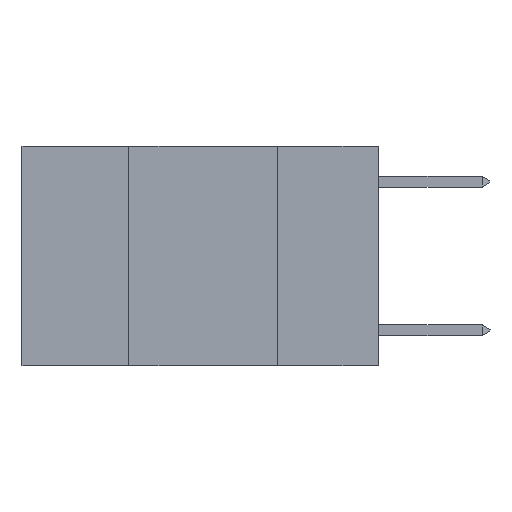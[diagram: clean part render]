
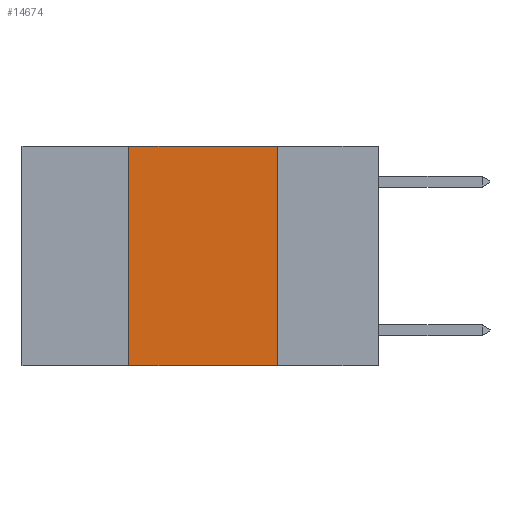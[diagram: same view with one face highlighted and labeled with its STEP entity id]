
A CAD part, left-side view. The second image highlights one B-rep face of the part: STEP entity #14674.
In plain terms, the highlighted planar face has unit normal (-1, 0, 0).
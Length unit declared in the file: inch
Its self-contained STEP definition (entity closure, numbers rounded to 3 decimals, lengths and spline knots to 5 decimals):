
#2302 = ORIENTED_EDGE ( 'NONE', *, *, #11323, .F. ) ;
#2516 = CARTESIAN_POINT ( 'NONE',  ( 0., 0.42, -0.37 ) ) ;
#2889 = VECTOR ( 'NONE', #8701, 39.37008 ) ;
#4548 = EDGE_CURVE ( 'NONE', #9651, #17047, #11353, .T. ) ;
#4781 = VECTOR ( 'NONE', #13084, 39.37008 ) ;
#5238 = DIRECTION ( 'NONE',  ( 0., 0., -1. ) ) ;
#6014 = EDGE_CURVE ( 'NONE', #7529, #14678, #7711, .T. ) ;
#6835 = CARTESIAN_POINT ( 'NONE',  ( 0., 0.17, -0.37 ) ) ;
#6923 = CARTESIAN_POINT ( 'NONE',  ( 0., 0.6, -0.37 ) ) ;
#7529 = VERTEX_POINT ( 'NONE', #2516 ) ;
#7711 = LINE ( 'NONE', #7807, #16832 ) ;
#7807 = CARTESIAN_POINT ( 'NONE',  ( 0., 0.42, 0. ) ) ;
#8701 = DIRECTION ( 'NONE',  ( 0., -1., 0. ) ) ;
#8879 = ORIENTED_EDGE ( 'NONE', *, *, #4548, .F. ) ;
#9391 = EDGE_CURVE ( 'NONE', #7529, #17047, #17040, .T. ) ;
#9634 = EDGE_LOOP ( 'NONE', ( #8879, #2302, #17890, #10650 ) ) ;
#9651 = VERTEX_POINT ( 'NONE', #10568 ) ;
#9659 = VECTOR ( 'NONE', #9911, 39.37008 ) ;
#9813 = CARTESIAN_POINT ( 'NONE',  ( 0., 0.17, 0. ) ) ;
#9911 = DIRECTION ( 'NONE',  ( 0., -1., 0. ) ) ;
#10568 = CARTESIAN_POINT ( 'NONE',  ( 0., 0.17, 0. ) ) ;
#10650 = ORIENTED_EDGE ( 'NONE', *, *, #9391, .T. ) ;
#10736 = FACE_OUTER_BOUND ( 'NONE', #9634, .T. ) ;
#11323 = EDGE_CURVE ( 'NONE', #14678, #9651, #11979, .T. ) ;
#11353 = LINE ( 'NONE', #9813, #4781 ) ;
#11979 = LINE ( 'NONE', #16297, #2889 ) ;
#12283 = CARTESIAN_POINT ( 'NONE',  ( 0., 0.42, 0. ) ) ;
#12349 = DIRECTION ( 'NONE',  ( 0., 0., 1. ) ) ;
#13084 = DIRECTION ( 'NONE',  ( 0., 0., -1. ) ) ;
#14011 = CARTESIAN_POINT ( 'NONE',  ( 0., 0.6, 0. ) ) ;
#14674 = ADVANCED_FACE ( 'NONE', ( #10736 ), #18441, .F. ) ;
#14678 = VERTEX_POINT ( 'NONE', #12283 ) ;
#16297 = CARTESIAN_POINT ( 'NONE',  ( 0., 0.6, 0. ) ) ;
#16832 = VECTOR ( 'NONE', #12349, 39.37008 ) ;
#17040 = LINE ( 'NONE', #6923, #9659 ) ;
#17047 = VERTEX_POINT ( 'NONE', #6835 ) ;
#17369 = AXIS2_PLACEMENT_3D ( 'NONE', #14011, #18248, #5238 ) ;
#17890 = ORIENTED_EDGE ( 'NONE', *, *, #6014, .F. ) ;
#18248 = DIRECTION ( 'NONE',  ( 1., 0., 0. ) ) ;
#18441 = PLANE ( 'NONE',  #17369 ) ;
